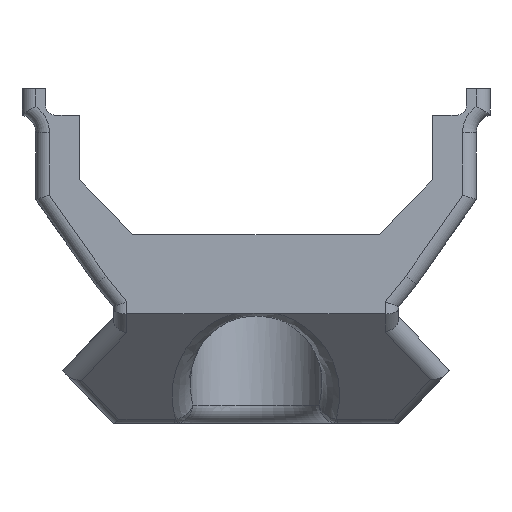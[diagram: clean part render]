
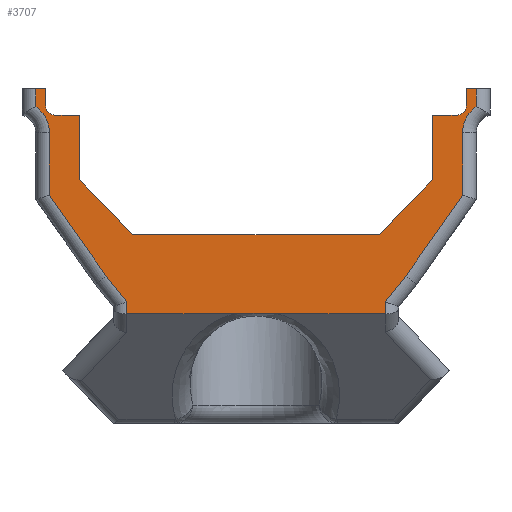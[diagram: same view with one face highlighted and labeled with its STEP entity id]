
A CAD part, front view. The second image highlights one B-rep face of the part: STEP entity #3707.
In plain terms, the highlighted planar face has unit normal (0, -1, 0).
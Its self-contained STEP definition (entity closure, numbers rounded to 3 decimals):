
#235=B_SPLINE_CURVE_WITH_KNOTS('',3,(#6746,#6747,#6748,#6749,#6750,#6751,
#6752,#6753,#6754,#6755,#6756,#6757,#6758,#6759,#6760,#6761,#6762,#6763),
 .UNSPECIFIED.,.F.,.F.,(4,2,2,2,2,2,2,2,4),(0.,0.064,0.086,
0.098,0.108,0.121,0.142,
0.186,0.205),.UNSPECIFIED.);
#335=PLANE('',#4038);
#524=FACE_OUTER_BOUND('',#717,.T.);
#717=EDGE_LOOP('',(#3433,#3434,#3435,#3436,#3437,#3438,#3439,#3440,#3441,
#3442,#3443,#3444,#3445,#3446,#3447,#3448,#3449,#3450,#3451,#3452,#3453,
#3454,#3455,#3456,#3457,#3458,#3459,#3460));
#757=LINE('',#5273,#1066);
#796=LINE('',#5956,#1105);
#808=LINE('',#6412,#1117);
#811=LINE('',#6418,#1120);
#814=LINE('',#6423,#1123);
#838=LINE('',#6789,#1147);
#856=LINE('',#6834,#1165);
#862=LINE('',#6861,#1171);
#864=LINE('',#6882,#1173);
#865=LINE('',#6889,#1174);
#867=LINE('',#6895,#1176);
#869=LINE('',#6901,#1178);
#876=LINE('',#6922,#1185);
#877=LINE('',#6925,#1186);
#878=LINE('',#6929,#1187);
#880=LINE('',#6954,#1189);
#934=LINE('',#7064,#1243);
#939=LINE('',#7079,#1248);
#944=LINE('',#7093,#1253);
#948=LINE('',#7102,#1257);
#1024=LINE('',#7261,#1333);
#1025=LINE('',#7263,#1334);
#1026=LINE('',#7265,#1335);
#1066=VECTOR('',#4151,10.);
#1105=VECTOR('',#4316,10.);
#1117=VECTOR('',#4444,10.);
#1120=VECTOR('',#4449,10.);
#1123=VECTOR('',#4454,10.);
#1147=VECTOR('',#4530,10.);
#1165=VECTOR('',#4572,10.);
#1171=VECTOR('',#4600,10.);
#1173=VECTOR('',#4606,10.);
#1174=VECTOR('',#4617,10.);
#1176=VECTOR('',#4623,10.);
#1178=VECTOR('',#4629,10.);
#1185=VECTOR('',#4654,10.);
#1186=VECTOR('',#4657,10.);
#1187=VECTOR('',#4662,10.);
#1189=VECTOR('',#4674,10.);
#1243=VECTOR('',#4756,10.);
#1248=VECTOR('',#4769,10.);
#1253=VECTOR('',#4782,10.);
#1257=VECTOR('',#4792,10.);
#1333=VECTOR('',#4976,10.);
#1334=VECTOR('',#4979,10.);
#1335=VECTOR('',#4982,10.);
#1393=CIRCLE('',#3933,1.75);
#1397=CIRCLE('',#3955,1.75);
#1400=CIRCLE('',#3972,0.5);
#1402=CIRCLE('',#3976,0.5);
#1479=VERTEX_POINT('',#5270);
#1480=VERTEX_POINT('',#5272);
#1568=VERTEX_POINT('',#5953);
#1569=VERTEX_POINT('',#5955);
#1601=VERTEX_POINT('',#6411);
#1603=VERTEX_POINT('',#6417);
#1633=VERTEX_POINT('',#6744);
#1634=VERTEX_POINT('',#6745);
#1643=VERTEX_POINT('',#6788);
#1657=VERTEX_POINT('',#6831);
#1658=VERTEX_POINT('',#6833);
#1667=VERTEX_POINT('',#6858);
#1668=VERTEX_POINT('',#6860);
#1670=VERTEX_POINT('',#6879);
#1671=VERTEX_POINT('',#6881);
#1672=VERTEX_POINT('',#6888);
#1674=VERTEX_POINT('',#6894);
#1676=VERTEX_POINT('',#6900);
#1682=VERTEX_POINT('',#6924);
#1683=VERTEX_POINT('',#6928);
#1686=VERTEX_POINT('',#6936);
#1687=VERTEX_POINT('',#6953);
#1729=VERTEX_POINT('',#7063);
#1731=VERTEX_POINT('',#7069);
#1732=VERTEX_POINT('',#7070);
#1735=VERTEX_POINT('',#7078);
#1737=VERTEX_POINT('',#7084);
#1738=VERTEX_POINT('',#7085);
#1854=EDGE_CURVE('',#1479,#1480,#757,.T.);
#1980=EDGE_CURVE('',#1569,#1568,#796,.T.);
#2048=EDGE_CURVE('',#1568,#1601,#808,.T.);
#2051=EDGE_CURVE('',#1601,#1603,#811,.T.);
#2054=EDGE_CURVE('',#1480,#1603,#814,.T.);
#2093=EDGE_CURVE('',#1633,#1634,#235,.T.);
#2107=EDGE_CURVE('',#1634,#1643,#838,.T.);
#2130=EDGE_CURVE('',#1657,#1658,#856,.T.);
#2143=EDGE_CURVE('',#1667,#1668,#862,.T.);
#2147=EDGE_CURVE('',#1670,#1671,#864,.T.);
#2149=EDGE_CURVE('',#1668,#1670,#1393,.T.);
#2151=EDGE_CURVE('',#1671,#1672,#865,.T.);
#2154=EDGE_CURVE('',#1672,#1674,#867,.T.);
#2157=EDGE_CURVE('',#1674,#1676,#869,.T.);
#2169=EDGE_CURVE('',#1643,#1657,#876,.T.);
#2170=EDGE_CURVE('',#1658,#1682,#877,.T.);
#2172=EDGE_CURVE('',#1682,#1683,#878,.T.);
#2176=EDGE_CURVE('',#1683,#1686,#1397,.T.);
#2178=EDGE_CURVE('',#1686,#1687,#880,.T.);
#2234=EDGE_CURVE('',#1687,#1729,#934,.T.);
#2237=EDGE_CURVE('',#1731,#1732,#1400,.T.);
#2241=EDGE_CURVE('',#1735,#1732,#939,.T.);
#2244=EDGE_CURVE('',#1737,#1738,#1402,.T.);
#2248=EDGE_CURVE('',#1738,#1479,#944,.T.);
#2253=EDGE_CURVE('',#1676,#1633,#948,.T.);
#2332=EDGE_CURVE('',#1667,#1735,#1024,.T.);
#2333=EDGE_CURVE('',#1731,#1569,#1025,.T.);
#2334=EDGE_CURVE('',#1729,#1737,#1026,.T.);
#3433=ORIENTED_EDGE('',*,*,#2093,.F.);
#3434=ORIENTED_EDGE('',*,*,#2253,.F.);
#3435=ORIENTED_EDGE('',*,*,#2157,.F.);
#3436=ORIENTED_EDGE('',*,*,#2154,.F.);
#3437=ORIENTED_EDGE('',*,*,#2151,.F.);
#3438=ORIENTED_EDGE('',*,*,#2147,.F.);
#3439=ORIENTED_EDGE('',*,*,#2149,.F.);
#3440=ORIENTED_EDGE('',*,*,#2143,.F.);
#3441=ORIENTED_EDGE('',*,*,#2332,.T.);
#3442=ORIENTED_EDGE('',*,*,#2241,.T.);
#3443=ORIENTED_EDGE('',*,*,#2237,.F.);
#3444=ORIENTED_EDGE('',*,*,#2333,.T.);
#3445=ORIENTED_EDGE('',*,*,#1980,.T.);
#3446=ORIENTED_EDGE('',*,*,#2048,.T.);
#3447=ORIENTED_EDGE('',*,*,#2051,.T.);
#3448=ORIENTED_EDGE('',*,*,#2054,.F.);
#3449=ORIENTED_EDGE('',*,*,#1854,.F.);
#3450=ORIENTED_EDGE('',*,*,#2248,.F.);
#3451=ORIENTED_EDGE('',*,*,#2244,.F.);
#3452=ORIENTED_EDGE('',*,*,#2334,.F.);
#3453=ORIENTED_EDGE('',*,*,#2234,.F.);
#3454=ORIENTED_EDGE('',*,*,#2178,.F.);
#3455=ORIENTED_EDGE('',*,*,#2176,.F.);
#3456=ORIENTED_EDGE('',*,*,#2172,.F.);
#3457=ORIENTED_EDGE('',*,*,#2170,.F.);
#3458=ORIENTED_EDGE('',*,*,#2130,.F.);
#3459=ORIENTED_EDGE('',*,*,#2169,.F.);
#3460=ORIENTED_EDGE('',*,*,#2107,.F.);
#3707=ADVANCED_FACE('',(#524),#335,.F.);
#3933=AXIS2_PLACEMENT_3D('',#6885,#4611,#4612);
#3955=AXIS2_PLACEMENT_3D('',#6937,#4670,#4671);
#3972=AXIS2_PLACEMENT_3D('',#7071,#4761,#4762);
#3976=AXIS2_PLACEMENT_3D('',#7086,#4774,#4775);
#4038=AXIS2_PLACEMENT_3D('',#7266,#4983,#4984);
#4151=DIRECTION('',(0.,0.,-1.));
#4316=DIRECTION('',(0.,0.,-1.));
#4444=DIRECTION('',(-0.696,0.,-0.718));
#4449=DIRECTION('',(-1.,0.,0.));
#4454=DIRECTION('',(0.696,0.,-0.718));
#4530=DIRECTION('',(-1.,0.,0.));
#4572=DIRECTION('',(-0.624,0.,0.782));
#4600=DIRECTION('',(0.,0.,-1.));
#4606=DIRECTION('',(0.,0.,-1.));
#4611=DIRECTION('center_axis',(0.,-1.,0.));
#4612=DIRECTION('ref_axis',(-0.791,0.,0.612));
#4617=DIRECTION('',(-0.575,0.,-0.818));
#4623=DIRECTION('',(-0.624,0.,-0.782));
#4629=DIRECTION('',(0.,0.,-1.));
#4654=DIRECTION('',(0.,0.,1.));
#4657=DIRECTION('',(-0.575,0.,0.818));
#4662=DIRECTION('',(0.,0.,1.));
#4670=DIRECTION('center_axis',(0.,-1.,0.));
#4671=DIRECTION('ref_axis',(0.791,0.,0.612));
#4674=DIRECTION('',(0.,0.,1.));
#4756=DIRECTION('',(1.,0.,0.));
#4761=DIRECTION('center_axis',(0.,-1.,0.));
#4762=DIRECTION('ref_axis',(0.707,0.,-0.707));
#4769=DIRECTION('',(0.,0.,-1.));
#4774=DIRECTION('center_axis',(0.,-1.,0.));
#4775=DIRECTION('ref_axis',(-0.707,0.,-0.707));
#4782=DIRECTION('',(1.,0.,0.));
#4792=DIRECTION('',(-1.,0.,0.));
#4976=DIRECTION('',(-1.,0.,0.));
#4979=DIRECTION('',(-1.,0.,0.));
#4982=DIRECTION('',(0.,0.,-1.));
#4983=DIRECTION('center_axis',(0.,1.,0.));
#4984=DIRECTION('ref_axis',(1.,0.,0.));
#5270=CARTESIAN_POINT('',(3.15,0.,11.9));
#5272=CARTESIAN_POINT('',(3.15,0.,8.35));
#5273=CARTESIAN_POINT('',(3.15,0.,11.9));
#5953=CARTESIAN_POINT('',(22.5,0.,8.35));
#5955=CARTESIAN_POINT('',(22.5,0.,11.9));
#5956=CARTESIAN_POINT('',(22.5,0.,11.9));
#6411=CARTESIAN_POINT('',(19.575,0.,5.336));
#6412=CARTESIAN_POINT('',(22.5,0.,8.35));
#6417=CARTESIAN_POINT('',(6.075,0.,5.336));
#6418=CARTESIAN_POINT('',(19.575,0.,5.336));
#6423=CARTESIAN_POINT('',(3.15,0.,8.35));
#6744=CARTESIAN_POINT('',(14.017,0.,1.006));
#6745=CARTESIAN_POINT('',(11.633,0.,1.006));
#6746=CARTESIAN_POINT('Ctrl Pts',(14.017,0.,
1.006));
#6747=CARTESIAN_POINT('Ctrl Pts',(13.802,0.,
1.006));
#6748=CARTESIAN_POINT('Ctrl Pts',(13.565,0.,
1.018));
#6749=CARTESIAN_POINT('Ctrl Pts',(13.211,0.,
1.029));
#6750=CARTESIAN_POINT('Ctrl Pts',(13.126,0.,
1.031));
#6751=CARTESIAN_POINT('Ctrl Pts',(12.989,0.,1.034));
#6752=CARTESIAN_POINT('Ctrl Pts',(12.939,0.,
1.034));
#6753=CARTESIAN_POINT('Ctrl Pts',(12.845,0.,
1.035));
#6754=CARTESIAN_POINT('Ctrl Pts',(12.802,0.,
1.035));
#6755=CARTESIAN_POINT('Ctrl Pts',(12.708,0.,
1.034));
#6756=CARTESIAN_POINT('Ctrl Pts',(12.658,0.,
1.034));
#6757=CARTESIAN_POINT('Ctrl Pts',(12.519,0.,
1.031));
#6758=CARTESIAN_POINT('Ctrl Pts',(12.433,0.,
1.029));
#6759=CARTESIAN_POINT('Ctrl Pts',(12.162,0.,
1.02));
#6760=CARTESIAN_POINT('Ctrl Pts',(11.998,0.,
1.013));
#6761=CARTESIAN_POINT('Ctrl Pts',(11.771,0.,
1.007));
#6762=CARTESIAN_POINT('Ctrl Pts',(11.701,0.,
1.006));
#6763=CARTESIAN_POINT('Ctrl Pts',(11.633,0.,
1.006));
#6788=CARTESIAN_POINT('',(5.739,0.,1.006));
#6789=CARTESIAN_POINT('',(16.743,0.,1.006));
#6831=CARTESIAN_POINT('',(5.739,0.,1.667));
#6833=CARTESIAN_POINT('',(4.619,0.,3.071));
#6834=CARTESIAN_POINT('',(5.945,0.,1.41));
#6858=CARTESIAN_POINT('',(24.9,0.,13.35));
#6860=CARTESIAN_POINT('',(24.9,0.,12.368));
#6861=CARTESIAN_POINT('',(24.9,0.,10.219));
#6879=CARTESIAN_POINT('',(24.15,0.,10.932));
#6881=CARTESIAN_POINT('',(24.15,0.,7.509));
#6882=CARTESIAN_POINT('',(24.15,0.,9.494));
#6885=CARTESIAN_POINT('Origin',(25.9,0.,10.932));
#6888=CARTESIAN_POINT('',(21.031,0.,3.071));
#6889=CARTESIAN_POINT('',(22.247,0.,4.801));
#6894=CARTESIAN_POINT('',(19.911,0.,1.667));
#6895=CARTESIAN_POINT('',(20.421,0.,2.307));
#6900=CARTESIAN_POINT('',(19.911,0.,1.006));
#6901=CARTESIAN_POINT('',(19.911,0.,5.708));
#6922=CARTESIAN_POINT('',(5.739,0.,3.94));
#6924=CARTESIAN_POINT('',(1.5,0.,7.509));
#6925=CARTESIAN_POINT('',(5.037,0.,2.476));
#6928=CARTESIAN_POINT('',(1.5,0.,10.932));
#6929=CARTESIAN_POINT('',(1.5,0.,7.18));
#6936=CARTESIAN_POINT('',(0.75,0.,12.368));
#6937=CARTESIAN_POINT('Origin',(-0.25,0.,10.932));
#6953=CARTESIAN_POINT('',(0.75,0.,13.35));
#6954=CARTESIAN_POINT('',(0.75,0.,9.494));
#7063=CARTESIAN_POINT('',(1.3,0.,13.35));
#7064=CARTESIAN_POINT('',(0.,0.,13.35));
#7069=CARTESIAN_POINT('',(23.85,0.,11.9));
#7070=CARTESIAN_POINT('',(24.35,0.,12.4));
#7071=CARTESIAN_POINT('Origin',(23.85,0.,12.4));
#7078=CARTESIAN_POINT('',(24.35,0.,13.35));
#7079=CARTESIAN_POINT('',(24.35,0.,13.35));
#7084=CARTESIAN_POINT('',(1.3,0.,12.4));
#7085=CARTESIAN_POINT('',(1.8,0.,11.9));
#7086=CARTESIAN_POINT('Origin',(1.8,0.,12.4));
#7093=CARTESIAN_POINT('',(0.75,0.,11.9));
#7102=CARTESIAN_POINT('',(16.743,0.,1.006));
#7261=CARTESIAN_POINT('',(25.65,0.,13.35));
#7263=CARTESIAN_POINT('',(24.9,0.,11.9));
#7265=CARTESIAN_POINT('',(1.3,0.,13.35));
#7266=CARTESIAN_POINT('Origin',(12.825,0.,7.089));
